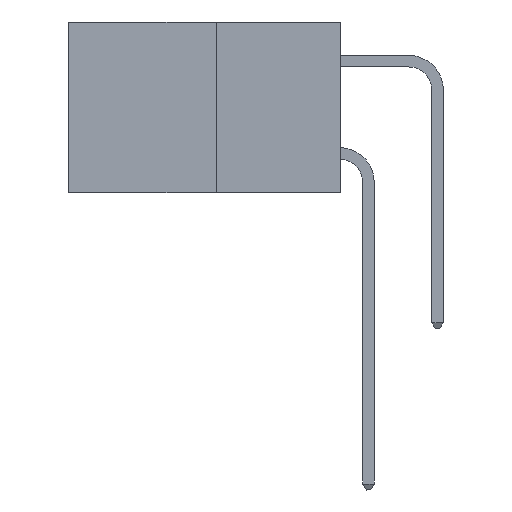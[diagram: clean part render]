
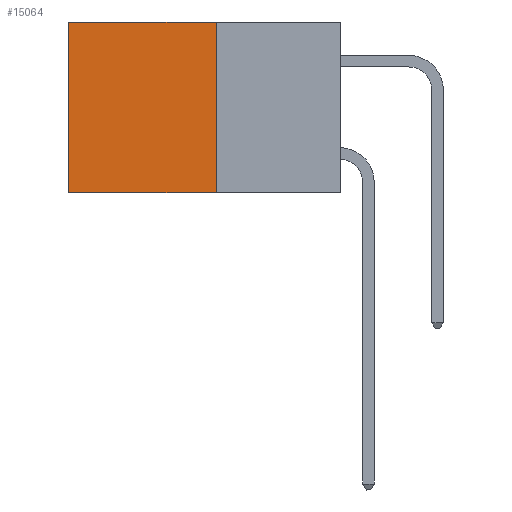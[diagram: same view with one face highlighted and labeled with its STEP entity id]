
A CAD part, left-side view. The second image highlights one B-rep face of the part: STEP entity #15064.
In plain terms, the highlighted planar face has unit normal (-1, 0, 0).
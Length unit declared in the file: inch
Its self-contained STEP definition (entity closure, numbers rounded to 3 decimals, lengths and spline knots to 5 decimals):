
#1647 = DIRECTION ( 'NONE',  ( 0., 1., 0. ) ) ;
#2881 = VECTOR ( 'NONE', #7570, 39.37008 ) ;
#3900 = CARTESIAN_POINT ( 'NONE',  ( 0.277, 0.27, 0. ) ) ;
#4485 = CARTESIAN_POINT ( 'NONE',  ( 0.277, 0.27, -0.37 ) ) ;
#4997 = CARTESIAN_POINT ( 'NONE',  ( 0.277, 0.27, -0.37 ) ) ;
#6245 = FACE_OUTER_BOUND ( 'NONE', #15625, .T. ) ;
#7072 = DIRECTION ( 'NONE',  ( 1., 0., 0. ) ) ;
#7570 = DIRECTION ( 'NONE',  ( 0., 0., -1. ) ) ;
#8335 = VECTOR ( 'NONE', #13088, 39.37008 ) ;
#9754 = VECTOR ( 'NONE', #11258, 39.37008 ) ;
#10304 = VERTEX_POINT ( 'NONE', #23453 ) ;
#10781 = VERTEX_POINT ( 'NONE', #28793 ) ;
#10836 = LINE ( 'NONE', #19544, #30305 ) ;
#11258 = DIRECTION ( 'NONE',  ( 0., 1., 0. ) ) ;
#13088 = DIRECTION ( 'NONE',  ( 0., 0., -1. ) ) ;
#15037 = ORIENTED_EDGE ( 'NONE', *, *, #16089, .T. ) ;
#15064 = ADVANCED_FACE ( 'NONE', ( #6245 ), #19756, .F. ) ;
#15561 = VERTEX_POINT ( 'NONE', #3900 ) ;
#15625 = EDGE_LOOP ( 'NONE', ( #30743, #16865, #25370, #15037 ) ) ;
#16089 = EDGE_CURVE ( 'NONE', #15561, #10304, #30029, .T. ) ;
#16865 = ORIENTED_EDGE ( 'NONE', *, *, #32835, .F. ) ;
#19544 = CARTESIAN_POINT ( 'NONE',  ( 0.277, 0.27, -0.37 ) ) ;
#19756 = PLANE ( 'NONE',  #23483 ) ;
#19968 = EDGE_CURVE ( 'NONE', #15561, #10781, #23254, .T. ) ;
#23254 = LINE ( 'NONE', #4997, #2881 ) ;
#23453 = CARTESIAN_POINT ( 'NONE',  ( 0.277, 0.59, 0. ) ) ;
#23483 = AXIS2_PLACEMENT_3D ( 'NONE', #4485, #7072, #24866 ) ;
#23927 = CARTESIAN_POINT ( 'NONE',  ( 0.277, 0.27, 0. ) ) ;
#24795 = EDGE_CURVE ( 'NONE', #10304, #28763, #28608, .T. ) ;
#24866 = DIRECTION ( 'NONE',  ( 0., 0., -1. ) ) ;
#25370 = ORIENTED_EDGE ( 'NONE', *, *, #19968, .F. ) ;
#25647 = CARTESIAN_POINT ( 'NONE',  ( 0.277, 0.59, -0.37 ) ) ;
#25792 = CARTESIAN_POINT ( 'NONE',  ( 0.277, 0.59, -0.37 ) ) ;
#28608 = LINE ( 'NONE', #25647, #8335 ) ;
#28763 = VERTEX_POINT ( 'NONE', #25792 ) ;
#28793 = CARTESIAN_POINT ( 'NONE',  ( 0.277, 0.27, -0.37 ) ) ;
#30029 = LINE ( 'NONE', #23927, #9754 ) ;
#30305 = VECTOR ( 'NONE', #1647, 39.37008 ) ;
#30743 = ORIENTED_EDGE ( 'NONE', *, *, #24795, .T. ) ;
#32835 = EDGE_CURVE ( 'NONE', #10781, #28763, #10836, .T. ) ;
